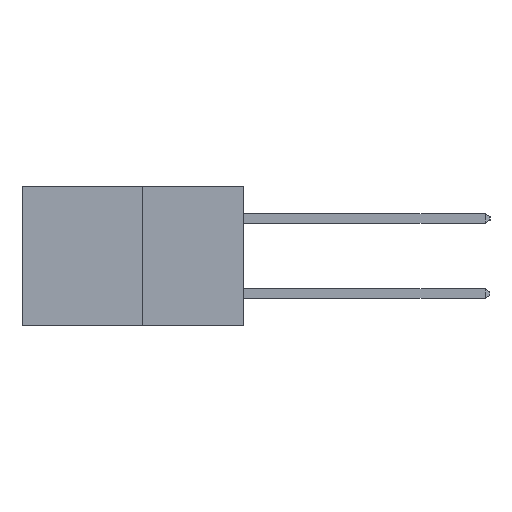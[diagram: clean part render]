
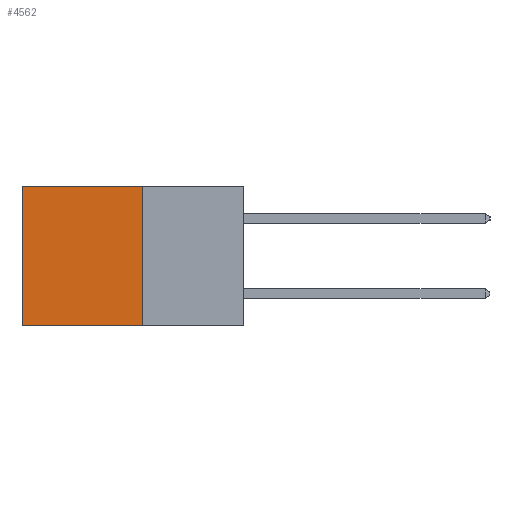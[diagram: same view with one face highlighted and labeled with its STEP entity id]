
A CAD part, left-side view. The second image highlights one B-rep face of the part: STEP entity #4562.
In plain terms, the highlighted planar face has unit normal (-1, 0, 0).
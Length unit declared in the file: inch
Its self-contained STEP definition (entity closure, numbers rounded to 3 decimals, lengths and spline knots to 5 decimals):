
#497 = FACE_OUTER_BOUND ( 'NONE', #16995, .T. ) ;
#824 = ORIENTED_EDGE ( 'NONE', *, *, #8655, .T. ) ;
#899 = CARTESIAN_POINT ( 'NONE',  ( 0.277, 0.59, -0.37 ) ) ;
#1690 = CARTESIAN_POINT ( 'NONE',  ( 0.277, 0.59, 0. ) ) ;
#2951 = VECTOR ( 'NONE', #18934, 39.37008 ) ;
#3047 = CARTESIAN_POINT ( 'NONE',  ( 0.277, 0.27, 0. ) ) ;
#3437 = VERTEX_POINT ( 'NONE', #1690 ) ;
#3596 = ORIENTED_EDGE ( 'NONE', *, *, #21669, .T. ) ;
#4562 = ADVANCED_FACE ( 'NONE', ( #497 ), #10943, .F. ) ;
#6180 = CARTESIAN_POINT ( 'NONE',  ( 0.277, 0.59, -0.37 ) ) ;
#6630 = CARTESIAN_POINT ( 'NONE',  ( 0.277, 0.27, -0.37 ) ) ;
#7505 = LINE ( 'NONE', #6630, #21387 ) ;
#8655 = EDGE_CURVE ( 'NONE', #15834, #3437, #19972, .T. ) ;
#9767 = CARTESIAN_POINT ( 'NONE',  ( 0.277, 0.27, -0.37 ) ) ;
#10393 = CARTESIAN_POINT ( 'NONE',  ( 0.277, 0.27, 0. ) ) ;
#10663 = DIRECTION ( 'NONE',  ( 0., 0., -1. ) ) ;
#10680 = DIRECTION ( 'NONE',  ( 1., 0., 0. ) ) ;
#10812 = CARTESIAN_POINT ( 'NONE',  ( 0.277, 0.27, -0.37 ) ) ;
#10943 = PLANE ( 'NONE',  #23365 ) ;
#11753 = CARTESIAN_POINT ( 'NONE',  ( 0.277, 0.27, -0.37 ) ) ;
#12217 = DIRECTION ( 'NONE',  ( 0., 1., 0. ) ) ;
#12662 = LINE ( 'NONE', #6180, #2951 ) ;
#13364 = ORIENTED_EDGE ( 'NONE', *, *, #13770, .F. ) ;
#13755 = LINE ( 'NONE', #9767, #23394 ) ;
#13770 = EDGE_CURVE ( 'NONE', #16928, #18166, #7505, .T. ) ;
#15139 = VECTOR ( 'NONE', #12217, 39.37008 ) ;
#15834 = VERTEX_POINT ( 'NONE', #10393 ) ;
#16633 = ORIENTED_EDGE ( 'NONE', *, *, #21602, .F. ) ;
#16928 = VERTEX_POINT ( 'NONE', #11753 ) ;
#16995 = EDGE_LOOP ( 'NONE', ( #3596, #13364, #16633, #824 ) ) ;
#18166 = VERTEX_POINT ( 'NONE', #899 ) ;
#18934 = DIRECTION ( 'NONE',  ( 0., 0., -1. ) ) ;
#19972 = LINE ( 'NONE', #3047, #15139 ) ;
#21119 = DIRECTION ( 'NONE',  ( 0., 1., 0. ) ) ;
#21387 = VECTOR ( 'NONE', #21119, 39.37008 ) ;
#21602 = EDGE_CURVE ( 'NONE', #15834, #16928, #13755, .T. ) ;
#21669 = EDGE_CURVE ( 'NONE', #3437, #18166, #12662, .T. ) ;
#22399 = DIRECTION ( 'NONE',  ( 0., 0., -1. ) ) ;
#23365 = AXIS2_PLACEMENT_3D ( 'NONE', #10812, #10680, #10663 ) ;
#23394 = VECTOR ( 'NONE', #22399, 39.37008 ) ;
